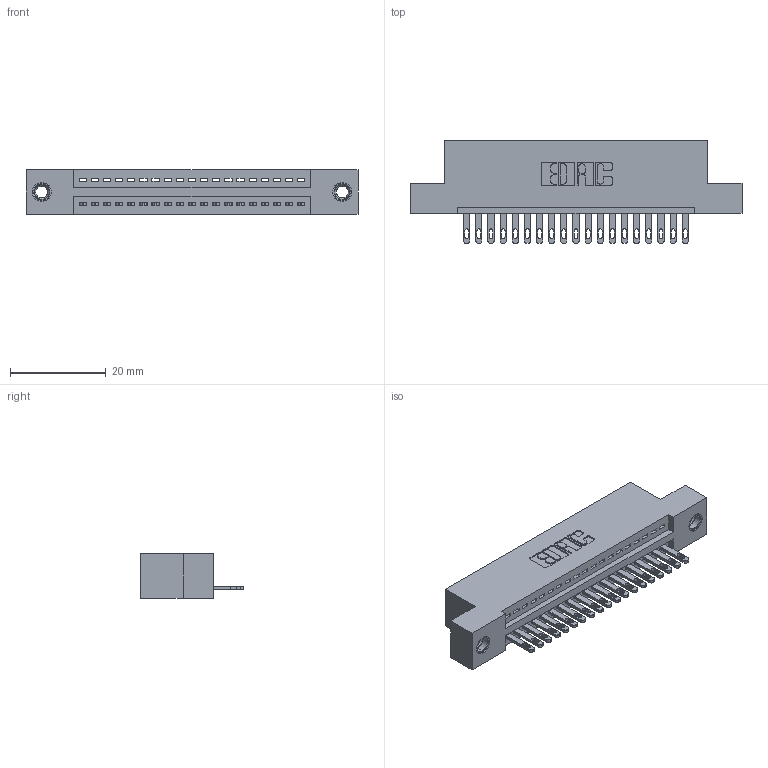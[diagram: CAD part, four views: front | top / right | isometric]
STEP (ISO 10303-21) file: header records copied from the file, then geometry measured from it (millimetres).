
FILE_DESCRIPTION (( 'STEP AP203' ), '1' );
FILE_NAME ('345-019-500-107.STEP', '2019-10-04T18:22:22', ( '' ), ( '' ), 'SwSTEP 2.0', 'SolidWorks 2016', '' );
FILE_SCHEMA (( 'CONFIG_CONTROL_DESIGN' ));
Length unit declared in the file: inch
Products named in the file (4): 345-292-001_345-293-100; 345 Part_Flush Mounting Lugs - 0.156 Dia-TI; 345-019-500-107; 345-250-001_345-250-005-103
Assembly tree (22 placements, depth 2):
  345-019-500-107
    345 Part_Flush Mounting Lugs - 0.156 Dia-TI
    345-292-001_345-293-100  x19
    345-250-001_345-250-005-103  x2
Bounding box: 69.47 x 21.51 x 9.4 mm (x, y, z)
Volume: 6408.1 mm3; surface area: 8278.4 mm2
Topology: 22 solids, 22 shells, 1212 faces, 3669 edges, 2438 vertices
Faces by surface type: plane 758, cylinder 438, cone 12, torus 4
Entity records: 18512 total; most frequent: CARTESIAN_POINT 3188, ORIENTED_EDGE 3134, DIRECTION 2847, EDGE_CURVE 1567, VECTOR 1335, LINE 1335, VERTEX_POINT 1040, AXIS2_PLACEMENT_3D 756
